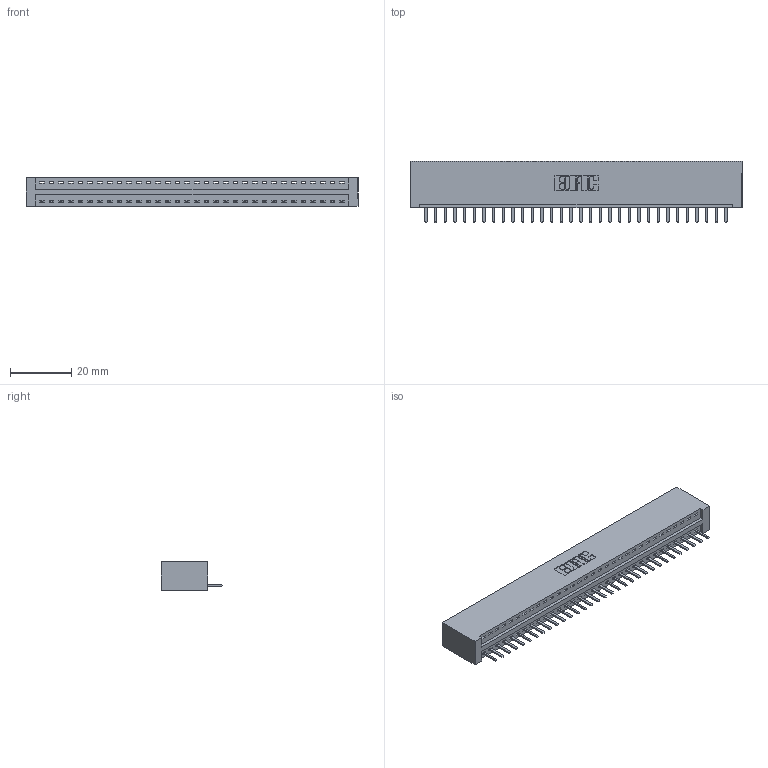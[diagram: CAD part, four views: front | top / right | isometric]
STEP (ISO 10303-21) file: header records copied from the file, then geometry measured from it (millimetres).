
FILE_DESCRIPTION (( 'STEP AP203' ), '1' );
FILE_NAME ('396-032-520-101.STEP', '2018-09-05T09:36:21', ( '' ), ( '' ), 'SwSTEP 2.0', 'SolidWorks 2016', '' );
FILE_SCHEMA (( 'CONFIG_CONTROL_DESIGN' ));
Length unit declared in the file: inch
Products named in the file (3): 346 Part_No Mounting Lugs; 345-292-001_345-293-120; 396-032-520-101
Assembly tree (33 placements, depth 2):
  396-032-520-101
    346 Part_No Mounting Lugs
    345-292-001_345-293-120  x32
Bounding box: 108.84 x 20.02 x 9.4 mm (x, y, z)
Volume: 10806.8 mm3; surface area: 13167 mm2
Topology: 33 solids, 33 shells, 2098 faces, 6193 edges, 4042 vertices
Faces by surface type: plane 1416, cylinder 682
Entity records: 21043 total; most frequent: CARTESIAN_POINT 3628, ORIENTED_EDGE 3582, DIRECTION 3195, EDGE_CURVE 1791, VECTOR 1535, LINE 1535, VERTEX_POINT 1190, AXIS2_PLACEMENT_3D 830
